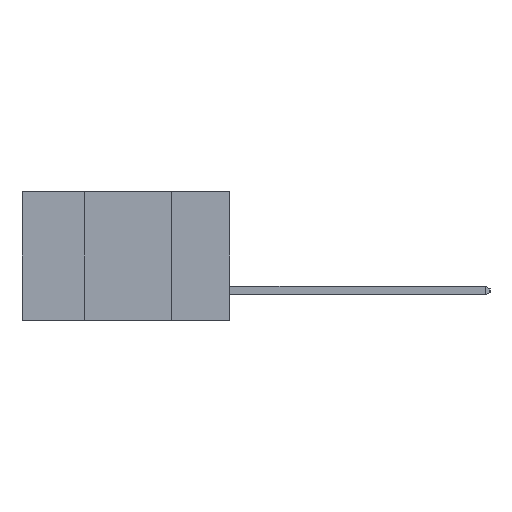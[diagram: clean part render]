
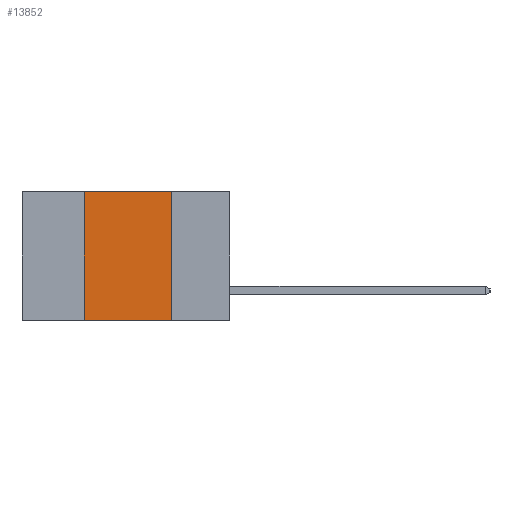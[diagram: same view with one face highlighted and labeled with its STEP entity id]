
A CAD part, left-side view. The second image highlights one B-rep face of the part: STEP entity #13852.
In plain terms, the highlighted planar face has unit normal (-1, 0, 0).
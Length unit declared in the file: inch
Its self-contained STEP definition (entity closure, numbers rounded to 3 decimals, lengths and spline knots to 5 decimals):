
#931 = ORIENTED_EDGE ( 'NONE', *, *, #15659, .F. ) ;
#1628 = DIRECTION ( 'NONE',  ( 0., 0., -1. ) ) ;
#2155 = CARTESIAN_POINT ( 'NONE',  ( 0., 0.42, 0. ) ) ;
#2481 = LINE ( 'NONE', #4866, #11043 ) ;
#2805 = AXIS2_PLACEMENT_3D ( 'NONE', #14380, #11312, #1628 ) ;
#4305 = CARTESIAN_POINT ( 'NONE',  ( 0., 0.17, 0. ) ) ;
#4710 = FACE_OUTER_BOUND ( 'NONE', #15879, .T. ) ;
#4866 = CARTESIAN_POINT ( 'NONE',  ( 0., 0.6, 0. ) ) ;
#5483 = CARTESIAN_POINT ( 'NONE',  ( 0., 0.42, -0.37 ) ) ;
#6512 = DIRECTION ( 'NONE',  ( 0., -1., 0. ) ) ;
#6611 = VERTEX_POINT ( 'NONE', #13139 ) ;
#8829 = VERTEX_POINT ( 'NONE', #5483 ) ;
#9051 = CARTESIAN_POINT ( 'NONE',  ( 0., 0.17, -0.37 ) ) ;
#10643 = ORIENTED_EDGE ( 'NONE', *, *, #13516, .F. ) ;
#11043 = VECTOR ( 'NONE', #6512, 39.37008 ) ;
#11312 = DIRECTION ( 'NONE',  ( 1., 0., 0. ) ) ;
#11361 = ORIENTED_EDGE ( 'NONE', *, *, #16712, .F. ) ;
#11478 = LINE ( 'NONE', #18651, #19239 ) ;
#12069 = CARTESIAN_POINT ( 'NONE',  ( 0., 0.42, -0.37 ) ) ;
#12475 = EDGE_CURVE ( 'NONE', #8829, #6611, #11478, .T. ) ;
#13139 = CARTESIAN_POINT ( 'NONE',  ( 0., 0.17, -0.37 ) ) ;
#13516 = EDGE_CURVE ( 'NONE', #8829, #17870, #19427, .T. ) ;
#13721 = DIRECTION ( 'NONE',  ( 0., 0., -1. ) ) ;
#13852 = ADVANCED_FACE ( 'NONE', ( #4710 ), #20505, .F. ) ;
#14380 = CARTESIAN_POINT ( 'NONE',  ( 0., 0.6, 0. ) ) ;
#15659 = EDGE_CURVE ( 'NONE', #17870, #19782, #2481, .T. ) ;
#15698 = VECTOR ( 'NONE', #13721, 39.37008 ) ;
#15879 = EDGE_LOOP ( 'NONE', ( #11361, #931, #10643, #15915 ) ) ;
#15915 = ORIENTED_EDGE ( 'NONE', *, *, #12475, .T. ) ;
#16198 = LINE ( 'NONE', #9051, #15698 ) ;
#16712 = EDGE_CURVE ( 'NONE', #19782, #6611, #16198, .T. ) ;
#17870 = VERTEX_POINT ( 'NONE', #2155 ) ;
#18355 = DIRECTION ( 'NONE',  ( 0., 0., 1. ) ) ;
#18651 = CARTESIAN_POINT ( 'NONE',  ( 0., 0.6, -0.37 ) ) ;
#18970 = VECTOR ( 'NONE', #18355, 39.37008 ) ;
#19239 = VECTOR ( 'NONE', #20104, 39.37008 ) ;
#19427 = LINE ( 'NONE', #12069, #18970 ) ;
#19782 = VERTEX_POINT ( 'NONE', #4305 ) ;
#20104 = DIRECTION ( 'NONE',  ( 0., -1., 0. ) ) ;
#20505 = PLANE ( 'NONE',  #2805 ) ;
